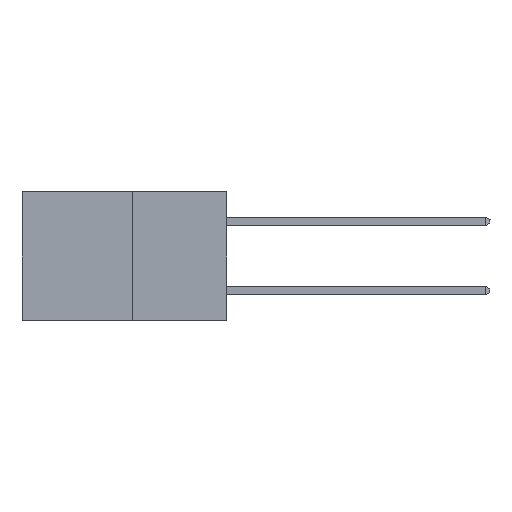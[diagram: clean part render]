
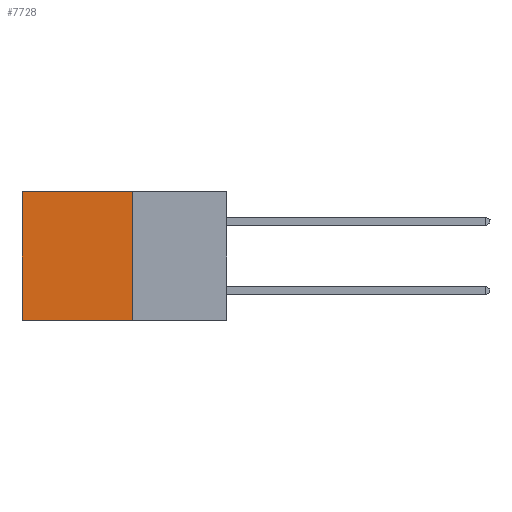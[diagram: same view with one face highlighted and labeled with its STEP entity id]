
A CAD part, left-side view. The second image highlights one B-rep face of the part: STEP entity #7728.
In plain terms, the highlighted planar face has unit normal (-1, 0, 0).
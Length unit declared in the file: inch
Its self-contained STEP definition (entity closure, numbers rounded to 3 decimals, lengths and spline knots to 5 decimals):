
#364 = ORIENTED_EDGE ( 'NONE', *, *, #4119, .F. ) ;
#766 = ORIENTED_EDGE ( 'NONE', *, *, #14963, .T. ) ;
#813 = PLANE ( 'NONE',  #13796 ) ;
#1662 = LINE ( 'NONE', #9658, #8091 ) ;
#1779 = VERTEX_POINT ( 'NONE', #15906 ) ;
#1874 = VERTEX_POINT ( 'NONE', #2444 ) ;
#2420 = FACE_OUTER_BOUND ( 'NONE', #9197, .T. ) ;
#2444 = CARTESIAN_POINT ( 'NONE',  ( 0.277, 0.59, -0.37 ) ) ;
#2701 = LINE ( 'NONE', #15752, #12495 ) ;
#2958 = EDGE_CURVE ( 'NONE', #1779, #1874, #6040, .T. ) ;
#3643 = VERTEX_POINT ( 'NONE', #15298 ) ;
#4119 = EDGE_CURVE ( 'NONE', #3643, #14341, #2701, .T. ) ;
#4720 = DIRECTION ( 'NONE',  ( 1., 0., 0. ) ) ;
#5021 = DIRECTION ( 'NONE',  ( 0., 0., -1. ) ) ;
#5501 = DIRECTION ( 'NONE',  ( 0., 0., -1. ) ) ;
#5628 = ORIENTED_EDGE ( 'NONE', *, *, #2958, .T. ) ;
#6040 = LINE ( 'NONE', #8494, #12330 ) ;
#6998 = EDGE_CURVE ( 'NONE', #14341, #1874, #1662, .T. ) ;
#7728 = ADVANCED_FACE ( 'NONE', ( #2420 ), #813, .F. ) ;
#8091 = VECTOR ( 'NONE', #10933, 39.37008 ) ;
#8494 = CARTESIAN_POINT ( 'NONE',  ( 0.277, 0.59, -0.37 ) ) ;
#9197 = EDGE_LOOP ( 'NONE', ( #5628, #9360, #364, #766 ) ) ;
#9360 = ORIENTED_EDGE ( 'NONE', *, *, #6998, .F. ) ;
#9658 = CARTESIAN_POINT ( 'NONE',  ( 0.277, 0.27, -0.37 ) ) ;
#10490 = VECTOR ( 'NONE', #12521, 39.37008 ) ;
#10933 = DIRECTION ( 'NONE',  ( 0., 1., 0. ) ) ;
#11250 = CARTESIAN_POINT ( 'NONE',  ( 0.277, 0.27, 0. ) ) ;
#12295 = CARTESIAN_POINT ( 'NONE',  ( 0.277, 0.27, -0.37 ) ) ;
#12330 = VECTOR ( 'NONE', #5501, 39.37008 ) ;
#12495 = VECTOR ( 'NONE', #5021, 39.37008 ) ;
#12521 = DIRECTION ( 'NONE',  ( 0., 1., 0. ) ) ;
#13503 = DIRECTION ( 'NONE',  ( 0., 0., -1. ) ) ;
#13795 = CARTESIAN_POINT ( 'NONE',  ( 0.277, 0.27, -0.37 ) ) ;
#13796 = AXIS2_PLACEMENT_3D ( 'NONE', #12295, #4720, #13503 ) ;
#14341 = VERTEX_POINT ( 'NONE', #13795 ) ;
#14520 = LINE ( 'NONE', #11250, #10490 ) ;
#14963 = EDGE_CURVE ( 'NONE', #3643, #1779, #14520, .T. ) ;
#15298 = CARTESIAN_POINT ( 'NONE',  ( 0.277, 0.27, 0. ) ) ;
#15752 = CARTESIAN_POINT ( 'NONE',  ( 0.277, 0.27, -0.37 ) ) ;
#15906 = CARTESIAN_POINT ( 'NONE',  ( 0.277, 0.59, 0. ) ) ;
